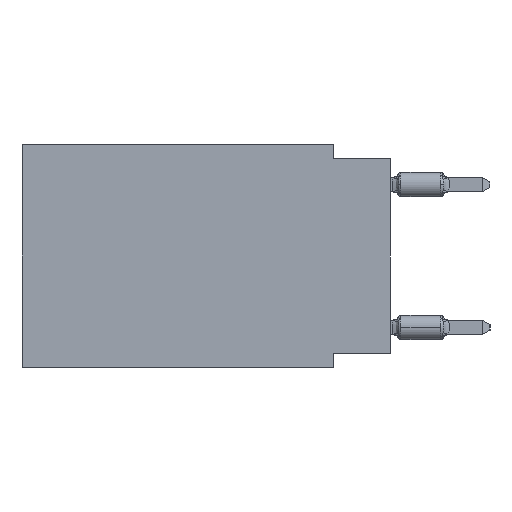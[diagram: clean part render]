
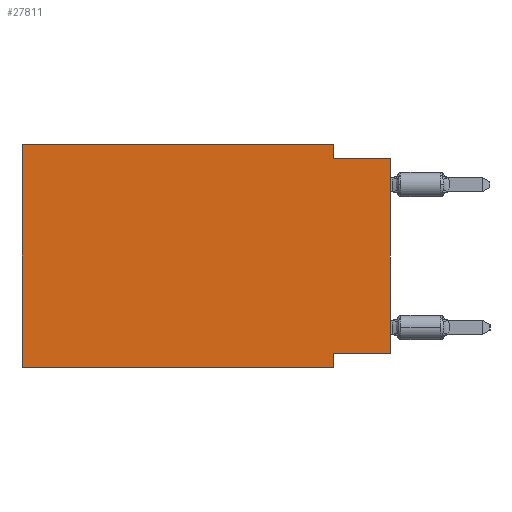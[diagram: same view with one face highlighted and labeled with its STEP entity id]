
A CAD part, left-side view. The second image highlights one B-rep face of the part: STEP entity #27811.
In plain terms, the highlighted planar face has unit normal (-1, 0, 0).
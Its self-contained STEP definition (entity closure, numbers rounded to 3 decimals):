
#117 = CARTESIAN_POINT ( 'NONE',  ( 0., 0., -9.271 ) ) ;
#1533 = CARTESIAN_POINT ( 'NONE',  ( 0., 16.383, -9.906 ) ) ;
#1957 = CARTESIAN_POINT ( 'NONE',  ( 0., 16.383, -9.906 ) ) ;
#2146 = CARTESIAN_POINT ( 'NONE',  ( 0., 16.383, 0. ) ) ;
#2213 = DIRECTION ( 'NONE',  ( 0., 0., -1. ) ) ;
#2695 = VECTOR ( 'NONE', #26063, 1000. ) ;
#2896 = ORIENTED_EDGE ( 'NONE', *, *, #37823, .F. ) ;
#3118 = CARTESIAN_POINT ( 'NONE',  ( 0., 2.54, 0. ) ) ;
#3164 = VERTEX_POINT ( 'NONE', #27818 ) ;
#4051 = VECTOR ( 'NONE', #5444, 1000. ) ;
#4398 = EDGE_CURVE ( 'NONE', #22836, #34738, #5769, .T. ) ;
#4932 = CARTESIAN_POINT ( 'NONE',  ( 0., 0., -0.635 ) ) ;
#5444 = DIRECTION ( 'NONE',  ( 0., 0., 1. ) ) ;
#5618 = ORIENTED_EDGE ( 'NONE', *, *, #31099, .F. ) ;
#5751 = DIRECTION ( 'NONE',  ( 0., -1., 0. ) ) ;
#5769 = LINE ( 'NONE', #37412, #32513 ) ;
#6201 = VERTEX_POINT ( 'NONE', #2146 ) ;
#7816 = ORIENTED_EDGE ( 'NONE', *, *, #17033, .T. ) ;
#8572 = LINE ( 'NONE', #31245, #4051 ) ;
#9372 = EDGE_CURVE ( 'NONE', #6201, #25848, #24789, .T. ) ;
#9745 = DIRECTION ( 'NONE',  ( 0., 0., 1. ) ) ;
#10321 = VERTEX_POINT ( 'NONE', #37594 ) ;
#11850 = DIRECTION ( 'NONE',  ( 1., 0., 0. ) ) ;
#11989 = CARTESIAN_POINT ( 'NONE',  ( 0., 0., -0.635 ) ) ;
#11990 = LINE ( 'NONE', #30730, #38630 ) ;
#12704 = CARTESIAN_POINT ( 'NONE',  ( 0., 16.383, 0. ) ) ;
#13065 = LINE ( 'NONE', #117, #31450 ) ;
#13359 = LINE ( 'NONE', #22330, #2695 ) ;
#13642 = DIRECTION ( 'NONE',  ( 0., -1., 0. ) ) ;
#13712 = EDGE_CURVE ( 'NONE', #20992, #10321, #13359, .T. ) ;
#14988 = PLANE ( 'NONE',  #37293 ) ;
#17033 = EDGE_CURVE ( 'NONE', #20476, #10321, #26943, .T. ) ;
#18642 = LINE ( 'NONE', #11989, #22786 ) ;
#18844 = VECTOR ( 'NONE', #13642, 1000. ) ;
#20053 = CARTESIAN_POINT ( 'NONE',  ( 0., 0., -9.271 ) ) ;
#20313 = EDGE_CURVE ( 'NONE', #22836, #20992, #13065, .T. ) ;
#20476 = VERTEX_POINT ( 'NONE', #1957 ) ;
#20992 = VERTEX_POINT ( 'NONE', #30812 ) ;
#22330 = CARTESIAN_POINT ( 'NONE',  ( 0., 2.54, -9.906 ) ) ;
#22786 = VECTOR ( 'NONE', #5751, 1000. ) ;
#22836 = VERTEX_POINT ( 'NONE', #20053 ) ;
#23181 = ORIENTED_EDGE ( 'NONE', *, *, #27343, .F. ) ;
#24789 = LINE ( 'NONE', #12704, #35645 ) ;
#25848 = VERTEX_POINT ( 'NONE', #3118 ) ;
#26063 = DIRECTION ( 'NONE',  ( 0., 0., -1. ) ) ;
#26384 = ORIENTED_EDGE ( 'NONE', *, *, #9372, .F. ) ;
#26943 = LINE ( 'NONE', #1533, #18844 ) ;
#27343 = EDGE_CURVE ( 'NONE', #20476, #6201, #8572, .T. ) ;
#27811 = ADVANCED_FACE ( 'NONE', ( #37457 ), #14988, .F. ) ;
#27818 = CARTESIAN_POINT ( 'NONE',  ( 0., 2.54, -0.635 ) ) ;
#28296 = CARTESIAN_POINT ( 'NONE',  ( 0., 16.383, 0. ) ) ;
#29067 = DIRECTION ( 'NONE',  ( 0., 1., 0. ) ) ;
#30256 = ORIENTED_EDGE ( 'NONE', *, *, #20313, .F. ) ;
#30730 = CARTESIAN_POINT ( 'NONE',  ( 0., 2.54, 0. ) ) ;
#30812 = CARTESIAN_POINT ( 'NONE',  ( 0., 2.54, -9.271 ) ) ;
#31099 = EDGE_CURVE ( 'NONE', #3164, #34738, #18642, .T. ) ;
#31245 = CARTESIAN_POINT ( 'NONE',  ( 0., 16.383, 0. ) ) ;
#31450 = VECTOR ( 'NONE', #29067, 1000. ) ;
#31897 = ORIENTED_EDGE ( 'NONE', *, *, #4398, .T. ) ;
#32513 = VECTOR ( 'NONE', #9745, 1000. ) ;
#34148 = ORIENTED_EDGE ( 'NONE', *, *, #13712, .F. ) ;
#34160 = DIRECTION ( 'NONE',  ( 0., -1., 0. ) ) ;
#34738 = VERTEX_POINT ( 'NONE', #4932 ) ;
#35645 = VECTOR ( 'NONE', #34160, 1000. ) ;
#37150 = EDGE_LOOP ( 'NONE', ( #31897, #5618, #2896, #26384, #23181, #7816, #34148, #30256 ) ) ;
#37293 = AXIS2_PLACEMENT_3D ( 'NONE', #28296, #11850, #41005 ) ;
#37412 = CARTESIAN_POINT ( 'NONE',  ( 0., 0., 0. ) ) ;
#37457 = FACE_OUTER_BOUND ( 'NONE', #37150, .T. ) ;
#37594 = CARTESIAN_POINT ( 'NONE',  ( 0., 2.54, -9.906 ) ) ;
#37823 = EDGE_CURVE ( 'NONE', #25848, #3164, #11990, .T. ) ;
#38630 = VECTOR ( 'NONE', #2213, 1000. ) ;
#41005 = DIRECTION ( 'NONE',  ( 0., 0., -1. ) ) ;
